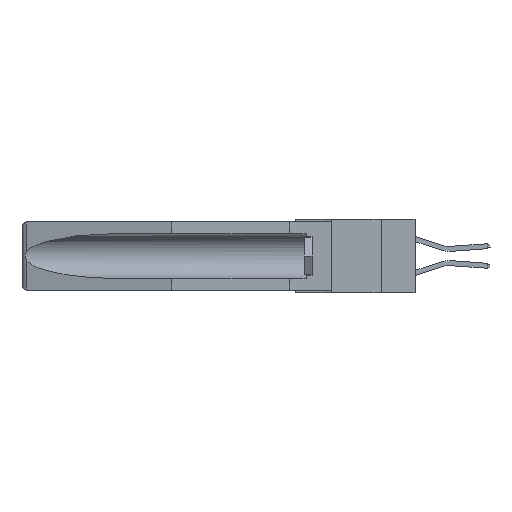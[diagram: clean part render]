
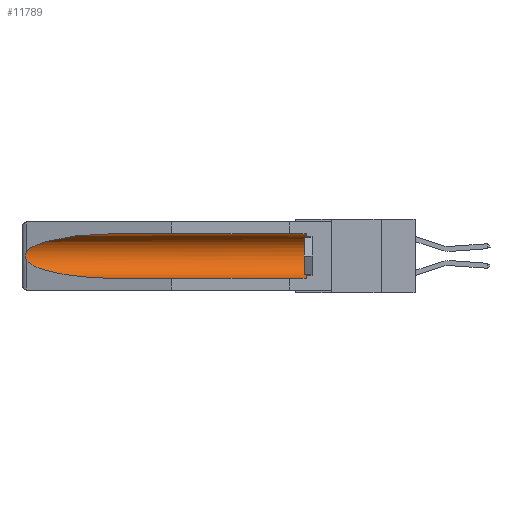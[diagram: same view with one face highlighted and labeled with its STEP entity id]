
A CAD part, left-side view. The second image highlights one B-rep face of the part: STEP entity #11789.
In plain terms, the highlighted cylindrical face has radius 2.857 mm (diameter 5.715 mm), a partial arc.
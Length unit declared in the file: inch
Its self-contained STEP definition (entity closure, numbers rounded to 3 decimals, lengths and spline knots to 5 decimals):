
#91 = CARTESIAN_POINT ( 'NONE',  ( 0.26537, 1.52718, -0.14972 ) ) ;
#598 = CARTESIAN_POINT ( 'NONE',  ( 0.26537, 1.52718, -0.19328 ) ) ;
#1272 =( BOUNDED_CURVE ( )  B_SPLINE_CURVE ( 3, ( #598, #21758, #15218, #3657 ),
 .UNSPECIFIED., .F., .F. ) 
 B_SPLINE_CURVE_WITH_KNOTS ( ( 4, 4 ),
 ( 0.1948, 1.5708 ),
 .UNSPECIFIED. ) 
 CURVE ( )  GEOMETRIC_REPRESENTATION_ITEM ( )  RATIONAL_B_SPLINE_CURVE ( ( 1., 0.848, 0.848, 1. ) ) 
 REPRESENTATION_ITEM ( '' )  );
#1859 = EDGE_CURVE ( 'NONE', #23299, #2271, #17084, .T. ) ;
#2212 = B_SPLINE_CURVE_WITH_KNOTS ( 'NONE', 3,
 ( #8218, #26849, #20041, #6112, #22384, #13008, #8116, #29274, #13100, #15456 ),
 .UNSPECIFIED., .F., .F.,
 ( 4, 2, 2, 2, 4 ),
 ( 0., 0.00029, 0.00058, 0.00087, 0.00117 ),
 .UNSPECIFIED. ) ;
#2271 = VERTEX_POINT ( 'NONE', #20075 ) ;
#2746 = DIRECTION ( 'NONE',  ( 0., 1., 0. ) ) ;
#3657 = CARTESIAN_POINT ( 'NONE',  ( 0.155, 1.07973, -0.284 ) ) ;
#5953 = LINE ( 'NONE', #8945, #9563 ) ;
#6112 = CARTESIAN_POINT ( 'NONE',  ( 0.2673, 1.5327, -0.16383 ) ) ;
#6706 = CARTESIAN_POINT ( 'NONE',  ( 0.155, 0.126, -0.284 ) ) ;
#7054 = CYLINDRICAL_SURFACE ( 'NONE', #10337, 0.1125 ) ;
#7112 = EDGE_CURVE ( 'NONE', #19846, #26723, #23823, .T. ) ;
#7161 = VERTEX_POINT ( 'NONE', #14318 ) ;
#8116 = CARTESIAN_POINT ( 'NONE',  ( 0.2673, 1.53269, -0.17917 ) ) ;
#8218 = CARTESIAN_POINT ( 'NONE',  ( 0.26537, 1.52718, -0.14972 ) ) ;
#8458 = ORIENTED_EDGE ( 'NONE', *, *, #26840, .T. ) ;
#8649 = DIRECTION ( 'NONE',  ( 0., 0., 1. ) ) ;
#8945 = CARTESIAN_POINT ( 'NONE',  ( 0.155, -0.30754, -0.059 ) ) ;
#9267 = EDGE_CURVE ( 'NONE', #26723, #7161, #2212, .T. ) ;
#9563 = VECTOR ( 'NONE', #22713, 39.37008 ) ;
#9624 = AXIS2_PLACEMENT_3D ( 'NONE', #11206, #11494, #8649 ) ;
#9850 = CARTESIAN_POINT ( 'NONE',  ( 0.155, -0.30754, -0.284 ) ) ;
#10337 = AXIS2_PLACEMENT_3D ( 'NONE', #21552, #2746, #23574 ) ;
#11206 = CARTESIAN_POINT ( 'NONE',  ( 0.155, 0.126, -0.1715 ) ) ;
#11494 = DIRECTION ( 'NONE',  ( 0., -1., 0. ) ) ;
#11789 = ADVANCED_FACE ( 'NONE', ( #23098 ), #7054, .F. ) ;
#13008 = CARTESIAN_POINT ( 'NONE',  ( 0.2675, 1.53308, -0.17534 ) ) ;
#13100 = CARTESIAN_POINT ( 'NONE',  ( 0.26597, 1.5296, -0.19026 ) ) ;
#14318 = CARTESIAN_POINT ( 'NONE',  ( 0.26537, 1.52718, -0.19328 ) ) ;
#15218 = CARTESIAN_POINT ( 'NONE',  ( 0.21114, 1.30732, -0.284 ) ) ;
#15456 = CARTESIAN_POINT ( 'NONE',  ( 0.26537, 1.52718, -0.19328 ) ) ;
#15473 = CARTESIAN_POINT ( 'NONE',  ( 0.21114, 1.30732, -0.059 ) ) ;
#15863 = ORIENTED_EDGE ( 'NONE', *, *, #20817, .T. ) ;
#16340 = EDGE_CURVE ( 'NONE', #23299, #26775, #23984, .T. ) ;
#16732 = VECTOR ( 'NONE', #23209, 39.37008 ) ;
#17084 = LINE ( 'NONE', #9850, #16732 ) ;
#17674 = ORIENTED_EDGE ( 'NONE', *, *, #16340, .T. ) ;
#19846 = VERTEX_POINT ( 'NONE', #22311 ) ;
#19876 = EDGE_LOOP ( 'NONE', ( #29379, #24478, #8458, #21195, #17674, #15863 ) ) ;
#20041 = CARTESIAN_POINT ( 'NONE',  ( 0.26654, 1.53092, -0.15636 ) ) ;
#20075 = CARTESIAN_POINT ( 'NONE',  ( 0.155, 1.07973, -0.284 ) ) ;
#20372 = CARTESIAN_POINT ( 'NONE',  ( 0.155, 1.07973, -0.059 ) ) ;
#20476 = CARTESIAN_POINT ( 'NONE',  ( 0.25451, 1.48313, -0.09465 ) ) ;
#20817 = EDGE_CURVE ( 'NONE', #26775, #19846, #5953, .T. ) ;
#21195 = ORIENTED_EDGE ( 'NONE', *, *, #1859, .F. ) ;
#21450 = CARTESIAN_POINT ( 'NONE',  ( 0.155, 0.126, -0.059 ) ) ;
#21552 = CARTESIAN_POINT ( 'NONE',  ( 0.155, -0.30754, -0.1715 ) ) ;
#21758 = CARTESIAN_POINT ( 'NONE',  ( 0.25451, 1.48313, -0.24835 ) ) ;
#22311 = CARTESIAN_POINT ( 'NONE',  ( 0.155, 1.07973, -0.059 ) ) ;
#22384 = CARTESIAN_POINT ( 'NONE',  ( 0.2675, 1.53308, -0.16763 ) ) ;
#22713 = DIRECTION ( 'NONE',  ( 0., 1., 0. ) ) ;
#23098 = FACE_OUTER_BOUND ( 'NONE', #19876, .T. ) ;
#23209 = DIRECTION ( 'NONE',  ( 0., 1., 0. ) ) ;
#23299 = VERTEX_POINT ( 'NONE', #6706 ) ;
#23574 = DIRECTION ( 'NONE',  ( 0., 0., 1. ) ) ;
#23823 =( BOUNDED_CURVE ( )  B_SPLINE_CURVE ( 3, ( #20372, #15473, #20476, #29596 ),
 .UNSPECIFIED., .F., .F. ) 
 B_SPLINE_CURVE_WITH_KNOTS ( ( 4, 4 ),
 ( 4.71239, 6.08839 ),
 .UNSPECIFIED. ) 
 CURVE ( )  GEOMETRIC_REPRESENTATION_ITEM ( )  RATIONAL_B_SPLINE_CURVE ( ( 1., 0.848, 0.848, 1. ) ) 
 REPRESENTATION_ITEM ( '' )  );
#23984 = CIRCLE ( 'NONE', #9624, 0.1125 ) ;
#24478 = ORIENTED_EDGE ( 'NONE', *, *, #9267, .T. ) ;
#26723 = VERTEX_POINT ( 'NONE', #91 ) ;
#26775 = VERTEX_POINT ( 'NONE', #21450 ) ;
#26840 = EDGE_CURVE ( 'NONE', #7161, #2271, #1272, .T. ) ;
#26849 = CARTESIAN_POINT ( 'NONE',  ( 0.26597, 1.52961, -0.15275 ) ) ;
#29274 = CARTESIAN_POINT ( 'NONE',  ( 0.26655, 1.53094, -0.18657 ) ) ;
#29379 = ORIENTED_EDGE ( 'NONE', *, *, #7112, .T. ) ;
#29596 = CARTESIAN_POINT ( 'NONE',  ( 0.26537, 1.52718, -0.14972 ) ) ;
